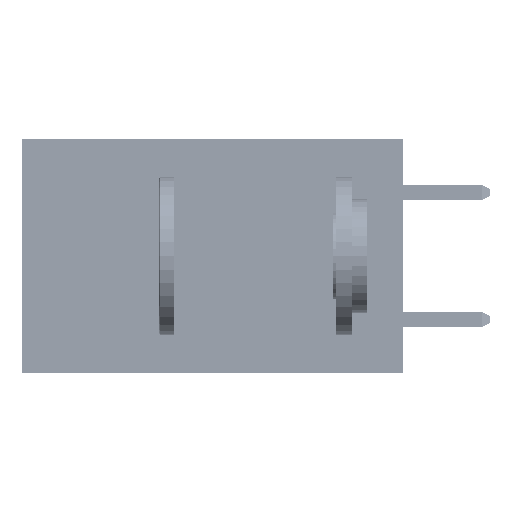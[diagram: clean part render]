
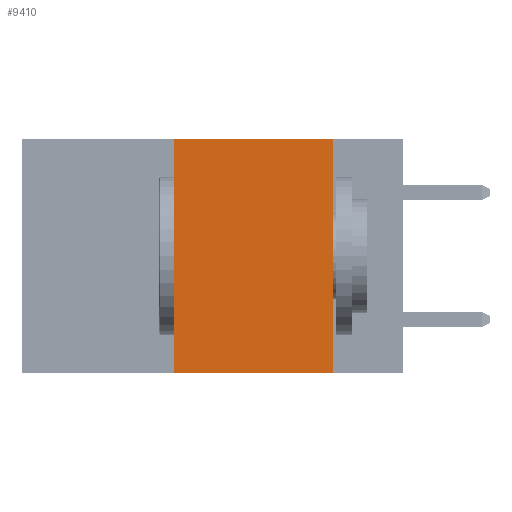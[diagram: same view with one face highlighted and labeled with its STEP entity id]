
A CAD part, left-side view. The second image highlights one B-rep face of the part: STEP entity #9410.
In plain terms, the highlighted planar face has unit normal (-1, 0, 0).
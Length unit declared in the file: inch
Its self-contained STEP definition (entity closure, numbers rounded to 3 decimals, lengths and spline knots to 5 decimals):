
#1358 = CARTESIAN_POINT ( 'NONE',  ( 0., 0.36, 0. ) ) ;
#2130 = DIRECTION ( 'NONE',  ( 0., 0., -1. ) ) ;
#2964 = CARTESIAN_POINT ( 'NONE',  ( 0., 0.11, -0.37 ) ) ;
#3266 = CARTESIAN_POINT ( 'NONE',  ( 0., 0.11, 0. ) ) ;
#3829 = LINE ( 'NONE', #9155, #28365 ) ;
#4114 = VECTOR ( 'NONE', #10375, 39.37008 ) ;
#5285 = DIRECTION ( 'NONE',  ( 0., 0., 1. ) ) ;
#5533 = PLANE ( 'NONE',  #21829 ) ;
#7381 = ORIENTED_EDGE ( 'NONE', *, *, #31183, .F. ) ;
#9155 = CARTESIAN_POINT ( 'NONE',  ( 0., 0.6, -0.37 ) ) ;
#9410 = ADVANCED_FACE ( 'NONE', ( #15996 ), #5533, .F. ) ;
#9750 = VERTEX_POINT ( 'NONE', #38768 ) ;
#10375 = DIRECTION ( 'NONE',  ( 0., 0., -1. ) ) ;
#11509 = CARTESIAN_POINT ( 'NONE',  ( 0., 0.6, 0. ) ) ;
#13314 = VECTOR ( 'NONE', #5285, 39.37008 ) ;
#13556 = VERTEX_POINT ( 'NONE', #43553 ) ;
#15996 = FACE_OUTER_BOUND ( 'NONE', #36133, .T. ) ;
#17722 = LINE ( 'NONE', #11509, #39802 ) ;
#17821 = CARTESIAN_POINT ( 'NONE',  ( 0., 0.6, 0. ) ) ;
#19453 = EDGE_CURVE ( 'NONE', #9750, #22389, #17722, .T. ) ;
#19990 = VERTEX_POINT ( 'NONE', #2964 ) ;
#21829 = AXIS2_PLACEMENT_3D ( 'NONE', #17821, #25069, #2130 ) ;
#22389 = VERTEX_POINT ( 'NONE', #28933 ) ;
#23125 = LINE ( 'NONE', #1358, #13314 ) ;
#24840 = ORIENTED_EDGE ( 'NONE', *, *, #19453, .F. ) ;
#25069 = DIRECTION ( 'NONE',  ( 1., 0., 0. ) ) ;
#28365 = VECTOR ( 'NONE', #34187, 39.37008 ) ;
#28933 = CARTESIAN_POINT ( 'NONE',  ( 0., 0.11, 0. ) ) ;
#31183 = EDGE_CURVE ( 'NONE', #13556, #9750, #23125, .T. ) ;
#34187 = DIRECTION ( 'NONE',  ( 0., -1., 0. ) ) ;
#35384 = LINE ( 'NONE', #3266, #4114 ) ;
#35681 = ORIENTED_EDGE ( 'NONE', *, *, #42287, .F. ) ;
#36133 = EDGE_LOOP ( 'NONE', ( #35681, #24840, #7381, #48797 ) ) ;
#37810 = EDGE_CURVE ( 'NONE', #13556, #19990, #3829, .T. ) ;
#38768 = CARTESIAN_POINT ( 'NONE',  ( 0., 0.36, 0. ) ) ;
#39802 = VECTOR ( 'NONE', #47567, 39.37008 ) ;
#42287 = EDGE_CURVE ( 'NONE', #22389, #19990, #35384, .T. ) ;
#43553 = CARTESIAN_POINT ( 'NONE',  ( 0., 0.36, -0.37 ) ) ;
#47567 = DIRECTION ( 'NONE',  ( 0., -1., 0. ) ) ;
#48797 = ORIENTED_EDGE ( 'NONE', *, *, #37810, .T. ) ;
